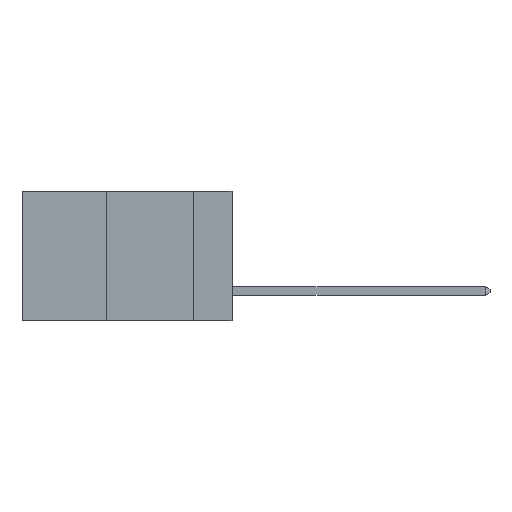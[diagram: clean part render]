
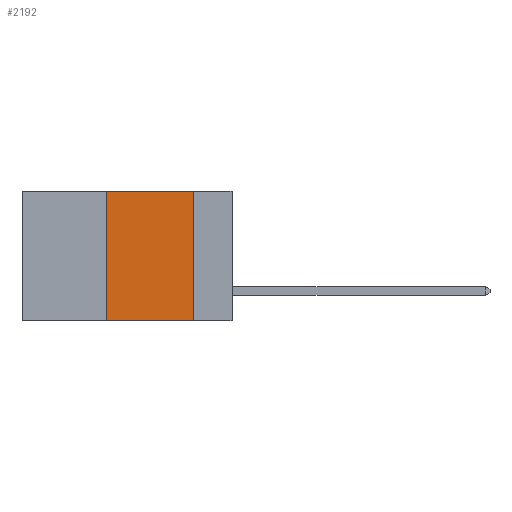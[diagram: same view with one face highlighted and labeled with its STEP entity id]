
A CAD part, left-side view. The second image highlights one B-rep face of the part: STEP entity #2192.
In plain terms, the highlighted planar face has unit normal (-1, 0, 0).
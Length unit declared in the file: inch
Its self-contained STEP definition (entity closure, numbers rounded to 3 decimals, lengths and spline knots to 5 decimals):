
#1193 = VERTEX_POINT ( 'NONE', #11422 ) ;
#1513 = PLANE ( 'NONE',  #7038 ) ;
#1739 = EDGE_CURVE ( 'NONE', #1193, #6797, #17129, .T. ) ;
#2192 = ADVANCED_FACE ( 'NONE', ( #17100 ), #1513, .F. ) ;
#3009 = VECTOR ( 'NONE', #23225, 39.37008 ) ;
#5569 = VECTOR ( 'NONE', #17026, 39.37008 ) ;
#6208 = ORIENTED_EDGE ( 'NONE', *, *, #25603, .F. ) ;
#6495 = DIRECTION ( 'NONE',  ( 0., -1., 0. ) ) ;
#6734 = CARTESIAN_POINT ( 'NONE',  ( 0., 0.6, 0. ) ) ;
#6797 = VERTEX_POINT ( 'NONE', #17117 ) ;
#6925 = DIRECTION ( 'NONE',  ( 1., 0., 0. ) ) ;
#7038 = AXIS2_PLACEMENT_3D ( 'NONE', #6734, #6925, #17323 ) ;
#7944 = EDGE_CURVE ( 'NONE', #6797, #9544, #13879, .T. ) ;
#8724 = VERTEX_POINT ( 'NONE', #16186 ) ;
#9544 = VERTEX_POINT ( 'NONE', #18927 ) ;
#9923 = DIRECTION ( 'NONE',  ( 0., -1., 0. ) ) ;
#11422 = CARTESIAN_POINT ( 'NONE',  ( 0., 0.36, 0. ) ) ;
#11625 = LINE ( 'NONE', #21191, #5569 ) ;
#11904 = ORIENTED_EDGE ( 'NONE', *, *, #1739, .F. ) ;
#12357 = EDGE_CURVE ( 'NONE', #8724, #9544, #17893, .T. ) ;
#13879 = LINE ( 'NONE', #25274, #3009 ) ;
#13988 = CARTESIAN_POINT ( 'NONE',  ( 0., 0.6, -0.37 ) ) ;
#16053 = ORIENTED_EDGE ( 'NONE', *, *, #7944, .F. ) ;
#16186 = CARTESIAN_POINT ( 'NONE',  ( 0., 0.36, -0.37 ) ) ;
#16456 = VECTOR ( 'NONE', #6495, 39.37008 ) ;
#17026 = DIRECTION ( 'NONE',  ( 0., 0., 1. ) ) ;
#17100 = FACE_OUTER_BOUND ( 'NONE', #22889, .T. ) ;
#17117 = CARTESIAN_POINT ( 'NONE',  ( 0., 0.11, 0. ) ) ;
#17129 = LINE ( 'NONE', #25829, #16456 ) ;
#17323 = DIRECTION ( 'NONE',  ( 0., 0., -1. ) ) ;
#17893 = LINE ( 'NONE', #13988, #22817 ) ;
#18927 = CARTESIAN_POINT ( 'NONE',  ( 0., 0.11, -0.37 ) ) ;
#21191 = CARTESIAN_POINT ( 'NONE',  ( 0., 0.36, 0. ) ) ;
#22817 = VECTOR ( 'NONE', #9923, 39.37008 ) ;
#22889 = EDGE_LOOP ( 'NONE', ( #16053, #11904, #6208, #26192 ) ) ;
#23225 = DIRECTION ( 'NONE',  ( 0., 0., -1. ) ) ;
#25274 = CARTESIAN_POINT ( 'NONE',  ( 0., 0.11, 0. ) ) ;
#25603 = EDGE_CURVE ( 'NONE', #8724, #1193, #11625, .T. ) ;
#25829 = CARTESIAN_POINT ( 'NONE',  ( 0., 0.6, 0. ) ) ;
#26192 = ORIENTED_EDGE ( 'NONE', *, *, #12357, .T. ) ;
